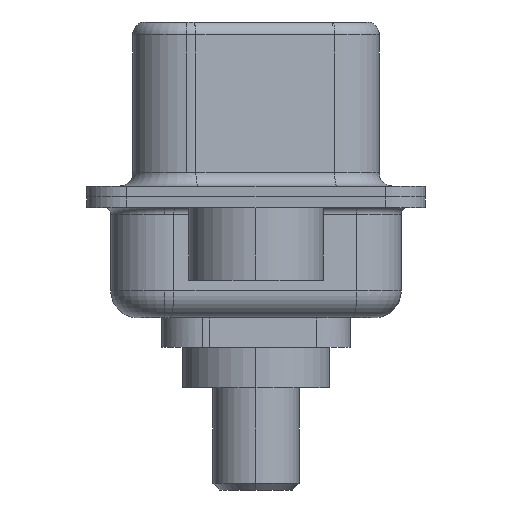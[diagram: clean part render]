
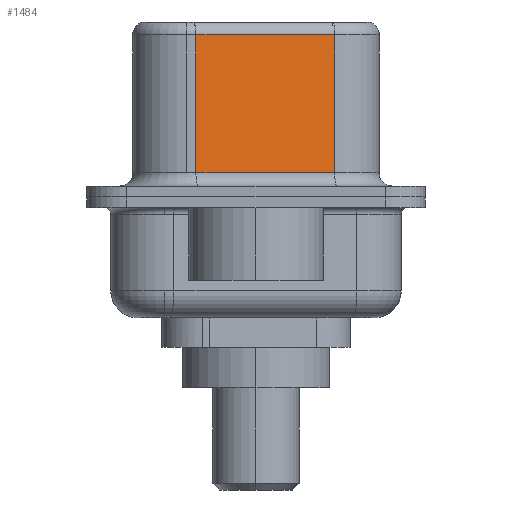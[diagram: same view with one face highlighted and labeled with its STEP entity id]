
A CAD part, left-side view. The second image highlights one B-rep face of the part: STEP entity #1484.
In plain terms, the highlighted planar face has unit normal (-0.985, -0.174, 0).
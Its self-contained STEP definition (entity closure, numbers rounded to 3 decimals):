
#225 = VECTOR ( 'NONE', #9534, 1000. ) ;
#1484 = ADVANCED_FACE ( 'NONE', ( #15302 ), #8980, .F. ) ;
#1699 = ORIENTED_EDGE ( 'NONE', *, *, #11242, .T. ) ;
#1848 = VERTEX_POINT ( 'NONE', #10348 ) ;
#2326 = VERTEX_POINT ( 'NONE', #6192 ) ;
#2729 = VECTOR ( 'NONE', #6329, 1000. ) ;
#2839 = CARTESIAN_POINT ( 'NONE',  ( 4.58, -2.927, 6.02 ) ) ;
#3042 = EDGE_CURVE ( 'NONE', #3357, #2326, #5981, .T. ) ;
#3334 = VECTOR ( 'NONE', #11044, 1000. ) ;
#3357 = VERTEX_POINT ( 'NONE', #6583 ) ;
#5066 = LINE ( 'NONE', #14606, #225 ) ;
#5980 = ORIENTED_EDGE ( 'NONE', *, *, #9118, .F. ) ;
#5981 = LINE ( 'NONE', #15999, #2729 ) ;
#6192 = CARTESIAN_POINT ( 'NONE',  ( 4.58, -2.927, 0.9 ) ) ;
#6329 = DIRECTION ( 'NONE',  ( 0.174, -0.985, 0. ) ) ;
#6456 = ORIENTED_EDGE ( 'NONE', *, *, #12365, .T. ) ;
#6583 = CARTESIAN_POINT ( 'NONE',  ( 3.67, 2.233, 0.9 ) ) ;
#7228 = VERTEX_POINT ( 'NONE', #2839 ) ;
#7668 = CARTESIAN_POINT ( 'NONE',  ( 4.58, -2.927, 6.52 ) ) ;
#8919 = DIRECTION ( 'NONE',  ( -0.174, 0.985, 0. ) ) ;
#8980 = PLANE ( 'NONE',  #15722 ) ;
#9085 = ORIENTED_EDGE ( 'NONE', *, *, #3042, .T. ) ;
#9118 = EDGE_CURVE ( 'NONE', #7228, #2326, #14193, .T. ) ;
#9459 = DIRECTION ( 'NONE',  ( -0.174, 0.985, 0. ) ) ;
#9534 = DIRECTION ( 'NONE',  ( 0., 0., -1. ) ) ;
#9774 = VECTOR ( 'NONE', #9459, 1000. ) ;
#10348 = CARTESIAN_POINT ( 'NONE',  ( 3.67, 2.233, 6.02 ) ) ;
#10560 = LINE ( 'NONE', #10654, #9774 ) ;
#10654 = CARTESIAN_POINT ( 'NONE',  ( 4.58, -2.927, 6.02 ) ) ;
#11044 = DIRECTION ( 'NONE',  ( 0., 0., -1. ) ) ;
#11242 = EDGE_CURVE ( 'NONE', #7228, #1848, #10560, .T. ) ;
#12365 = EDGE_CURVE ( 'NONE', #1848, #3357, #5066, .T. ) ;
#13947 = DIRECTION ( 'NONE',  ( 0.985, 0.174, 0. ) ) ;
#14193 = LINE ( 'NONE', #15942, #3334 ) ;
#14327 = EDGE_LOOP ( 'NONE', ( #5980, #1699, #6456, #9085 ) ) ;
#14606 = CARTESIAN_POINT ( 'NONE',  ( 3.67, 2.233, 6.52 ) ) ;
#15302 = FACE_OUTER_BOUND ( 'NONE', #14327, .T. ) ;
#15722 = AXIS2_PLACEMENT_3D ( 'NONE', #7668, #13947, #8919 ) ;
#15942 = CARTESIAN_POINT ( 'NONE',  ( 4.58, -2.927, 6.52 ) ) ;
#15999 = CARTESIAN_POINT ( 'NONE',  ( 4.58, -2.927, 0.9 ) ) ;
